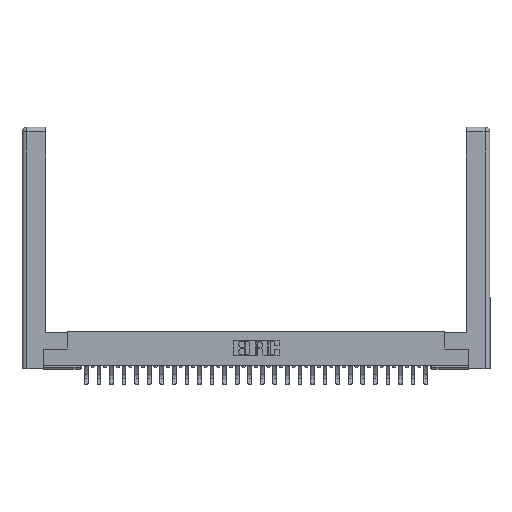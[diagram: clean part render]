
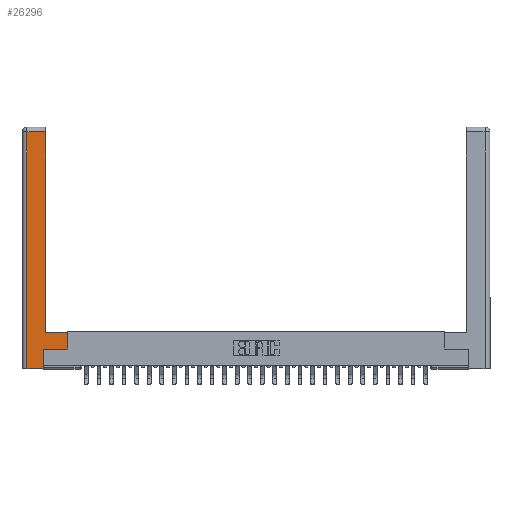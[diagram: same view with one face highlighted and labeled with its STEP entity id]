
A CAD part, top view. The second image highlights one B-rep face of the part: STEP entity #26296.
In plain terms, the highlighted planar face has unit normal (0, 0, 1).
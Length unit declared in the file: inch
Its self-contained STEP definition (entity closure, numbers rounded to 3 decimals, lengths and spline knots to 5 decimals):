
#659 = DIRECTION ( 'NONE',  ( 1., 0., 0. ) ) ;
#1255 = VERTEX_POINT ( 'NONE', #11344 ) ;
#1982 = LINE ( 'NONE', #4252, #5880 ) ;
#3565 = VECTOR ( 'NONE', #19773, 39.37008 ) ;
#4122 = ORIENTED_EDGE ( 'NONE', *, *, #6286, .T. ) ;
#4252 = CARTESIAN_POINT ( 'NONE',  ( 0.265, 0.245, 0. ) ) ;
#4554 = EDGE_CURVE ( 'NONE', #7832, #17404, #17258, .T. ) ;
#4597 = VECTOR ( 'NONE', #10579, 39.37008 ) ;
#4768 = CARTESIAN_POINT ( 'NONE',  ( 0.565, 0.45, 0. ) ) ;
#5880 = VECTOR ( 'NONE', #19891, 39.37008 ) ;
#6152 = CARTESIAN_POINT ( 'NONE',  ( 0.565, 0.245, 0. ) ) ;
#6249 = VECTOR ( 'NONE', #29255, 39.37008 ) ;
#6286 = EDGE_CURVE ( 'NONE', #16117, #16062, #21786, .T. ) ;
#6925 = EDGE_CURVE ( 'NONE', #17404, #1255, #16440, .T. ) ;
#7693 = CARTESIAN_POINT ( 'NONE',  ( 0.0615, 2.94, 0. ) ) ;
#7832 = VERTEX_POINT ( 'NONE', #10402 ) ;
#7880 = VECTOR ( 'NONE', #659, 39.37008 ) ;
#8255 = ORIENTED_EDGE ( 'NONE', *, *, #12638, .T. ) ;
#8286 = VECTOR ( 'NONE', #23733, 39.37008 ) ;
#8342 = VECTOR ( 'NONE', #13109, 39.37008 ) ;
#8628 = EDGE_LOOP ( 'NONE', ( #26467, #11616, #22060, #27802, #19941, #4122, #8255, #12975 ) ) ;
#9074 = LINE ( 'NONE', #4768, #16134 ) ;
#10402 = CARTESIAN_POINT ( 'NONE',  ( 0.295, 0.45, 0. ) ) ;
#10579 = DIRECTION ( 'NONE',  ( -1., 0., 0. ) ) ;
#11116 = CARTESIAN_POINT ( 'NONE',  ( 0.265, 0.245, 0. ) ) ;
#11344 = CARTESIAN_POINT ( 'NONE',  ( 0.0615, 2.94, 0. ) ) ;
#11616 = ORIENTED_EDGE ( 'NONE', *, *, #6925, .T. ) ;
#11733 = VERTEX_POINT ( 'NONE', #13166 ) ;
#11799 = DIRECTION ( 'NONE',  ( 0., 1., 0. ) ) ;
#12638 = EDGE_CURVE ( 'NONE', #16062, #11733, #9074, .T. ) ;
#12975 = ORIENTED_EDGE ( 'NONE', *, *, #24730, .T. ) ;
#13064 = CARTESIAN_POINT ( 'NONE',  ( 0.295, 0.45, 0. ) ) ;
#13109 = DIRECTION ( 'NONE',  ( 1., 0., 0. ) ) ;
#13166 = CARTESIAN_POINT ( 'NONE',  ( 0.565, 0.45, 0. ) ) ;
#13505 = LINE ( 'NONE', #17896, #3565 ) ;
#13927 = VERTEX_POINT ( 'NONE', #25890 ) ;
#14450 = EDGE_CURVE ( 'NONE', #20334, #13927, #18168, .T. ) ;
#16062 = VERTEX_POINT ( 'NONE', #22098 ) ;
#16117 = VERTEX_POINT ( 'NONE', #11116 ) ;
#16134 = VECTOR ( 'NONE', #11799, 39.37008 ) ;
#16440 = LINE ( 'NONE', #7693, #8286 ) ;
#17093 = CARTESIAN_POINT ( 'NONE',  ( 0.0615, 0., 0. ) ) ;
#17258 = LINE ( 'NONE', #29148, #6249 ) ;
#17404 = VERTEX_POINT ( 'NONE', #26801 ) ;
#17896 = CARTESIAN_POINT ( 'NONE',  ( 0.0615, 0., 0. ) ) ;
#18168 = LINE ( 'NONE', #21279, #7880 ) ;
#18588 = PLANE ( 'NONE',  #26055 ) ;
#18698 = EDGE_CURVE ( 'NONE', #13927, #16117, #1982, .T. ) ;
#18873 = DIRECTION ( 'NONE',  ( -1., 0., 0. ) ) ;
#19773 = DIRECTION ( 'NONE',  ( 0., -1., 0. ) ) ;
#19891 = DIRECTION ( 'NONE',  ( 0., 1., 0. ) ) ;
#19941 = ORIENTED_EDGE ( 'NONE', *, *, #18698, .T. ) ;
#20119 = FACE_OUTER_BOUND ( 'NONE', #8628, .T. ) ;
#20334 = VERTEX_POINT ( 'NONE', #17093 ) ;
#20748 = DIRECTION ( 'NONE',  ( 0., 0., -1. ) ) ;
#21242 = LINE ( 'NONE', #13064, #4597 ) ;
#21279 = CARTESIAN_POINT ( 'NONE',  ( 0.265, 0., 0. ) ) ;
#21786 = LINE ( 'NONE', #6152, #8342 ) ;
#22060 = ORIENTED_EDGE ( 'NONE', *, *, #22341, .T. ) ;
#22098 = CARTESIAN_POINT ( 'NONE',  ( 0.565, 0.245, 0. ) ) ;
#22341 = EDGE_CURVE ( 'NONE', #1255, #20334, #13505, .T. ) ;
#23413 = CARTESIAN_POINT ( 'NONE',  ( 0., 0., 0. ) ) ;
#23733 = DIRECTION ( 'NONE',  ( -1., 0., 0. ) ) ;
#24730 = EDGE_CURVE ( 'NONE', #11733, #7832, #21242, .T. ) ;
#25890 = CARTESIAN_POINT ( 'NONE',  ( 0.265, 0., 0. ) ) ;
#26055 = AXIS2_PLACEMENT_3D ( 'NONE', #23413, #20748, #18873 ) ;
#26296 = ADVANCED_FACE ( 'NONE', ( #20119 ), #18588, .F. ) ;
#26467 = ORIENTED_EDGE ( 'NONE', *, *, #4554, .T. ) ;
#26801 = CARTESIAN_POINT ( 'NONE',  ( 0.295, 2.94, 0. ) ) ;
#27802 = ORIENTED_EDGE ( 'NONE', *, *, #14450, .T. ) ;
#29148 = CARTESIAN_POINT ( 'NONE',  ( 0.295, 3., 0. ) ) ;
#29255 = DIRECTION ( 'NONE',  ( 0., 1., 0. ) ) ;
